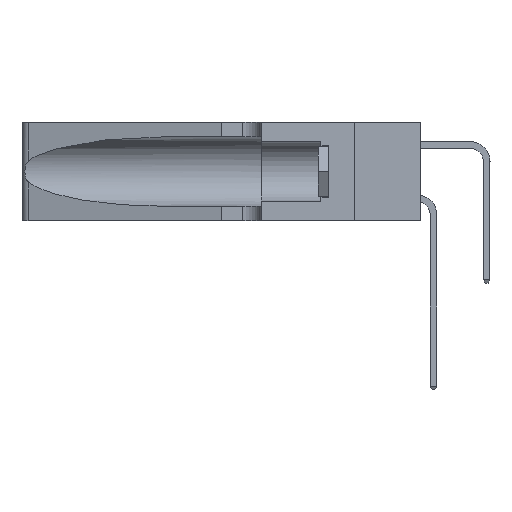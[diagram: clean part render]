
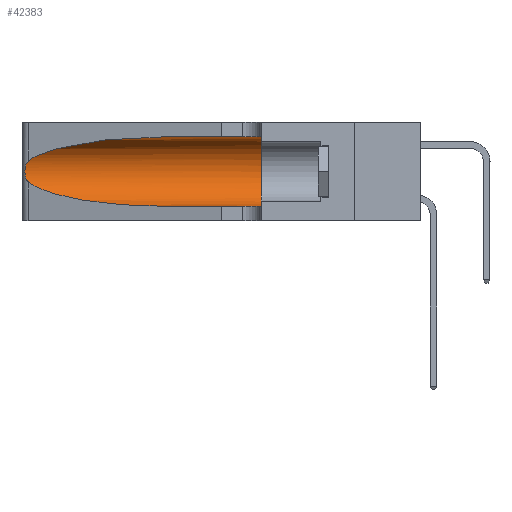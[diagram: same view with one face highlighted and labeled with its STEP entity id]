
A CAD part, left-side view. The second image highlights one B-rep face of the part: STEP entity #42383.
In plain terms, the highlighted cylindrical face has radius 3.308 mm (diameter 6.617 mm), a partial arc.
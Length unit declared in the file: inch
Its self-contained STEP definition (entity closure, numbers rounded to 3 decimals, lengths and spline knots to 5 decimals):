
#528 = ORIENTED_EDGE ( 'NONE', *, *, #19295, .T. ) ;
#2180 = CARTESIAN_POINT ( 'NONE',  ( 0.1305, 1.61858, 0.31525 ) ) ;
#2346 = CARTESIAN_POINT ( 'NONE',  ( 0.26075, 1.23896, 0.178 ) ) ;
#2607 = CARTESIAN_POINT ( 'NONE',  ( 0.1305, 0.72297, 0.05475 ) ) ;
#2809 = LINE ( 'NONE', #37106, #37778 ) ;
#4337 = CARTESIAN_POINT ( 'NONE',  ( 0.1305, 0.72297, 0.31525 ) ) ;
#4857 = CIRCLE ( 'NONE', #42790, 0.13025 ) ;
#5224 = VERTEX_POINT ( 'NONE', #29188 ) ;
#5755 = CARTESIAN_POINT ( 'NONE',  ( 0.25487, 1.22718, 0.22369 ) ) ;
#6147 = CARTESIAN_POINT ( 'NONE',  ( 0.25487, 1.22718, 0.14631 ) ) ;
#6264 = DIRECTION ( 'NONE',  ( 0., 1., 0. ) ) ;
#9116 = CARTESIAN_POINT ( 'NONE',  ( 0.25487, 1.22718, 0.14631 ) ) ;
#10178 = VERTEX_POINT ( 'NONE', #16058 ) ;
#11210 = ORIENTED_EDGE ( 'NONE', *, *, #42663, .T. ) ;
#12089 = CARTESIAN_POINT ( 'NONE',  ( 0.26018, 1.23835, 0.19895 ) ) ;
#14797 = EDGE_CURVE ( 'NONE', #5224, #10178, #42362, .T. ) ;
#16041 = CARTESIAN_POINT ( 'NONE',  ( 0.2373, 1.15595, 0.08982 ) ) ;
#16058 = CARTESIAN_POINT ( 'NONE',  ( 0.1305, 0.72297, 0.05475 ) ) ;
#17507 = CARTESIAN_POINT ( 'NONE',  ( 0.25487, 1.22718, 0.22369 ) ) ;
#17554 = FACE_OUTER_BOUND ( 'NONE', #42174, .T. ) ;
#18184 = VECTOR ( 'NONE', #25673, 39.37008 ) ;
#18714 = DIRECTION ( 'NONE',  ( 0., 0., -1. ) ) ;
#18718 = LINE ( 'NONE', #2180, #18184 ) ;
#19036 = CARTESIAN_POINT ( 'NONE',  ( 0.26017, 1.23833, 0.17102 ) ) ;
#19295 = EDGE_CURVE ( 'NONE', #42094, #5224, #27024, .T. ) ;
#21912 = EDGE_CURVE ( 'NONE', #28572, #34889, #18718, .T. ) ;
#22161 = CARTESIAN_POINT ( 'NONE',  ( 0.25856, 1.23593, 0.16098 ) ) ;
#22302 = CARTESIAN_POINT ( 'NONE',  ( 0.2373, 1.15595, 0.28018 ) ) ;
#22601 = CARTESIAN_POINT ( 'NONE',  ( 0.26075, 1.23896, 0.19203 ) ) ;
#22745 = CARTESIAN_POINT ( 'NONE',  ( 0.25787, 1.23484, 0.2124 ) ) ;
#22858 = CARTESIAN_POINT ( 'NONE',  ( 0.18966, 0.96281, 0.05475 ) ) ;
#22860 = ORIENTED_EDGE ( 'NONE', *, *, #24523, .F. ) ;
#23702 = EDGE_CURVE ( 'NONE', #28572, #42094, #40414, .T. ) ;
#24328 = AXIS2_PLACEMENT_3D ( 'NONE', #32644, #32789, #18714 ) ;
#24523 = EDGE_CURVE ( 'NONE', #34889, #36299, #4857, .T. ) ;
#25248 = CARTESIAN_POINT ( 'NONE',  ( 0.1305, 0.72297, 0.31525 ) ) ;
#25673 = DIRECTION ( 'NONE',  ( 0., -1., 0. ) ) ;
#25967 = CARTESIAN_POINT ( 'NONE',  ( 0.25639, 1.23186, 0.15144 ) ) ;
#27024 = B_SPLINE_CURVE_WITH_KNOTS ( 'NONE', 3,
 ( #5755, #36127, #39427, #22745, #32529, #12089, #22601, #2346, #19036, #22161, #42877, #25967, #29427, #9116 ),
 .UNSPECIFIED., .F., .F.,
 ( 4, 2, 2, 2, 2, 2, 4 ),
 ( 0., 0.00027, 0.00053, 0.00107, 0.0016, 0.00187, 0.00214 ),
 .UNSPECIFIED. ) ;
#27138 = ORIENTED_EDGE ( 'NONE', *, *, #23702, .T. ) ;
#28346 = ORIENTED_EDGE ( 'NONE', *, *, #14797, .T. ) ;
#28537 = CARTESIAN_POINT ( 'NONE',  ( 0.25487, 1.22718, 0.22369 ) ) ;
#28572 = VERTEX_POINT ( 'NONE', #4337 ) ;
#29188 = CARTESIAN_POINT ( 'NONE',  ( 0.25487, 1.22718, 0.14631 ) ) ;
#29320 = CYLINDRICAL_SURFACE ( 'NONE', #24328, 0.13025 ) ;
#29368 = ORIENTED_EDGE ( 'NONE', *, *, #21912, .F. ) ;
#29427 = CARTESIAN_POINT ( 'NONE',  ( 0.25555, 1.22993, 0.14849 ) ) ;
#32286 = CARTESIAN_POINT ( 'NONE',  ( 0.1305, 0.35, 0.31525 ) ) ;
#32529 = CARTESIAN_POINT ( 'NONE',  ( 0.25854, 1.2359, 0.20912 ) ) ;
#32644 = CARTESIAN_POINT ( 'NONE',  ( 0.1305, 1.61858, 0.185 ) ) ;
#32789 = DIRECTION ( 'NONE',  ( 0., -1., 0. ) ) ;
#33949 = DIRECTION ( 'NONE',  ( 0., -1., 0. ) ) ;
#34889 = VERTEX_POINT ( 'NONE', #32286 ) ;
#36127 = CARTESIAN_POINT ( 'NONE',  ( 0.25555, 1.22994, 0.2215 ) ) ;
#36299 = VERTEX_POINT ( 'NONE', #42075 ) ;
#37106 = CARTESIAN_POINT ( 'NONE',  ( 0.1305, 1.61858, 0.05475 ) ) ;
#37778 = VECTOR ( 'NONE', #33949, 39.37008 ) ;
#38955 = CARTESIAN_POINT ( 'NONE',  ( 0.18966, 0.96281, 0.31525 ) ) ;
#39427 = CARTESIAN_POINT ( 'NONE',  ( 0.25639, 1.23184, 0.21858 ) ) ;
#40232 = DIRECTION ( 'NONE',  ( 0., 0., 1. ) ) ;
#40414 =( BOUNDED_CURVE ( )  B_SPLINE_CURVE ( 3, ( #25248, #38955, #22302, #28537 ),
 .UNSPECIFIED., .F., .T. ) 
 B_SPLINE_CURVE_WITH_KNOTS ( ( 4, 4 ),
 ( 1.5708, 2.84003 ),
 .UNSPECIFIED. ) 
 CURVE ( )  GEOMETRIC_REPRESENTATION_ITEM ( )  RATIONAL_B_SPLINE_CURVE ( ( 1., 0.87, 0.87, 1. ) ) 
 REPRESENTATION_ITEM ( '' )  );
#42075 = CARTESIAN_POINT ( 'NONE',  ( 0.1305, 0.35, 0.05475 ) ) ;
#42094 = VERTEX_POINT ( 'NONE', #17507 ) ;
#42174 = EDGE_LOOP ( 'NONE', ( #27138, #528, #28346, #11210, #22860, #29368 ) ) ;
#42362 =( BOUNDED_CURVE ( )  B_SPLINE_CURVE ( 3, ( #6147, #16041, #22858, #2607 ),
 .UNSPECIFIED., .F., .T. ) 
 B_SPLINE_CURVE_WITH_KNOTS ( ( 4, 4 ),
 ( 3.44316, 4.71239 ),
 .UNSPECIFIED. ) 
 CURVE ( )  GEOMETRIC_REPRESENTATION_ITEM ( )  RATIONAL_B_SPLINE_CURVE ( ( 1., 0.87, 0.87, 1. ) ) 
 REPRESENTATION_ITEM ( '' )  );
#42383 = ADVANCED_FACE ( 'NONE', ( #17554 ), #29320, .F. ) ;
#42663 = EDGE_CURVE ( 'NONE', #10178, #36299, #2809, .T. ) ;
#42790 = AXIS2_PLACEMENT_3D ( 'NONE', #43397, #6264, #40232 ) ;
#42877 = CARTESIAN_POINT ( 'NONE',  ( 0.25789, 1.23486, 0.15765 ) ) ;
#43397 = CARTESIAN_POINT ( 'NONE',  ( 0.1305, 0.35, 0.185 ) ) ;
